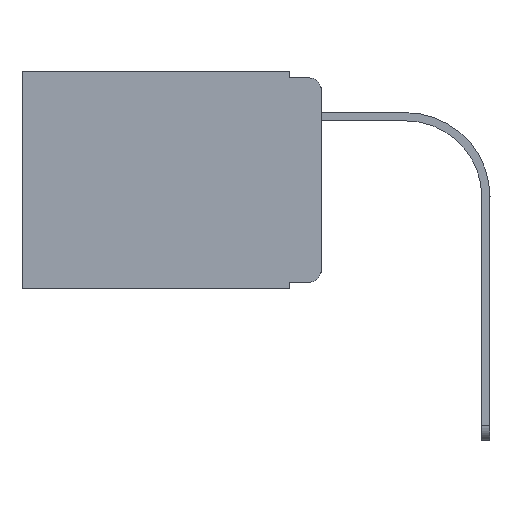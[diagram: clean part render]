
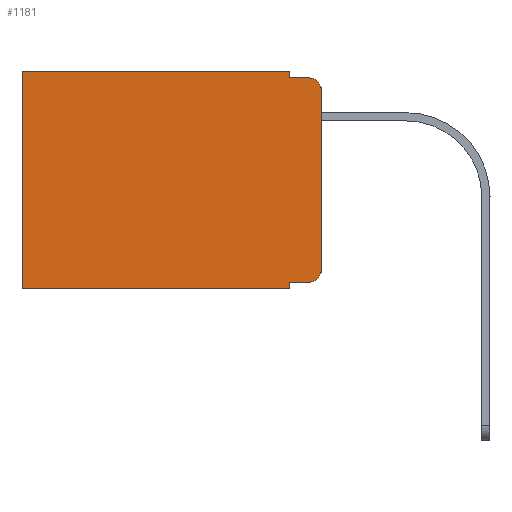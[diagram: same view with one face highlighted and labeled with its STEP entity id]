
A CAD part, left-side view. The second image highlights one B-rep face of the part: STEP entity #1181.
In plain terms, the highlighted planar face has unit normal (-1, 0, 0).
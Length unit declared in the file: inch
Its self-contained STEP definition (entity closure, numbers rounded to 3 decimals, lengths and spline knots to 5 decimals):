
#88 = DIRECTION ( 'NONE',  ( 0., 1., 0. ) ) ;
#89 = VERTEX_POINT ( 'NONE', #3949 ) ;
#189 = CARTESIAN_POINT ( 'NONE',  ( 0.298, 0., 0. ) ) ;
#239 = LINE ( 'NONE', #189, #3472 ) ;
#240 = ORIENTED_EDGE ( 'NONE', *, *, #1186, .T. ) ;
#448 = DIRECTION ( 'NONE',  ( 0., 0., -1. ) ) ;
#552 = EDGE_CURVE ( 'NONE', #5223, #10134, #5753, .T. ) ;
#951 = DIRECTION ( 'NONE',  ( -1., 0., 0. ) ) ;
#1024 = VERTEX_POINT ( 'NONE', #6915 ) ;
#1033 = FACE_OUTER_BOUND ( 'NONE', #5975, .T. ) ;
#1137 = ORIENTED_EDGE ( 'NONE', *, *, #7990, .T. ) ;
#1181 = ADVANCED_FACE ( 'NONE', ( #1033 ), #5618, .F. ) ;
#1186 = EDGE_CURVE ( 'NONE', #3363, #9292, #239, .T. ) ;
#1256 = VERTEX_POINT ( 'NONE', #2739 ) ;
#1648 = VERTEX_POINT ( 'NONE', #8376 ) ;
#1734 = VECTOR ( 'NONE', #4858, 39.37008 ) ;
#1932 = CARTESIAN_POINT ( 'NONE',  ( 0.298, 0.051, -0.333 ) ) ;
#2245 = CARTESIAN_POINT ( 'NONE',  ( 0.298, 0., 0. ) ) ;
#2311 = LINE ( 'NONE', #7768, #10085 ) ;
#2401 = VECTOR ( 'NONE', #448, 39.37008 ) ;
#2627 = CIRCLE ( 'NONE', #2946, 0.02 ) ;
#2739 = CARTESIAN_POINT ( 'NONE',  ( 0.298, 0.051, -0.343 ) ) ;
#2856 = CARTESIAN_POINT ( 'NONE',  ( 0.298, 0.473, 0. ) ) ;
#2946 = AXIS2_PLACEMENT_3D ( 'NONE', #3174, #951, #6260 ) ;
#3081 = CARTESIAN_POINT ( 'NONE',  ( 0.298, 0.02, -0.313 ) ) ;
#3103 = ORIENTED_EDGE ( 'NONE', *, *, #4603, .F. ) ;
#3139 = DIRECTION ( 'NONE',  ( 0., -1., 0. ) ) ;
#3174 = CARTESIAN_POINT ( 'NONE',  ( 0.298, 0.02, -0.03 ) ) ;
#3324 = AXIS2_PLACEMENT_3D ( 'NONE', #4110, #3389, #7936 ) ;
#3363 = VERTEX_POINT ( 'NONE', #3829 ) ;
#3389 = DIRECTION ( 'NONE',  ( 1., 0., 0. ) ) ;
#3392 = ORIENTED_EDGE ( 'NONE', *, *, #9044, .F. ) ;
#3472 = VECTOR ( 'NONE', #88, 39.37008 ) ;
#3829 = CARTESIAN_POINT ( 'NONE',  ( 0.298, 0.051, 0. ) ) ;
#3929 = VECTOR ( 'NONE', #8483, 39.37008 ) ;
#3949 = CARTESIAN_POINT ( 'NONE',  ( 0.298, 0., -0.03 ) ) ;
#4045 = CARTESIAN_POINT ( 'NONE',  ( 0.298, 0.051, -0.01 ) ) ;
#4110 = CARTESIAN_POINT ( 'NONE',  ( 0.298, 0., 0. ) ) ;
#4142 = LINE ( 'NONE', #8029, #1734 ) ;
#4181 = ORIENTED_EDGE ( 'NONE', *, *, #8760, .F. ) ;
#4237 = AXIS2_PLACEMENT_3D ( 'NONE', #3081, #7598, #8438 ) ;
#4336 = CARTESIAN_POINT ( 'NONE',  ( 0.298, 0.02, -0.333 ) ) ;
#4603 = EDGE_CURVE ( 'NONE', #5223, #1256, #7674, .T. ) ;
#4723 = VECTOR ( 'NONE', #7966, 39.37008 ) ;
#4814 = ORIENTED_EDGE ( 'NONE', *, *, #7805, .T. ) ;
#4858 = DIRECTION ( 'NONE',  ( 0., 0., -1. ) ) ;
#5137 = EDGE_CURVE ( 'NONE', #1648, #5416, #9325, .T. ) ;
#5188 = EDGE_CURVE ( 'NONE', #1256, #9279, #2311, .T. ) ;
#5223 = VERTEX_POINT ( 'NONE', #1932 ) ;
#5351 = CARTESIAN_POINT ( 'NONE',  ( 0.298, 0.02, -0.01 ) ) ;
#5413 = DIRECTION ( 'NONE',  ( 0., 1., 0. ) ) ;
#5416 = VERTEX_POINT ( 'NONE', #5351 ) ;
#5487 = VECTOR ( 'NONE', #3139, 39.37008 ) ;
#5618 = PLANE ( 'NONE',  #3324 ) ;
#5753 = LINE ( 'NONE', #9616, #4723 ) ;
#5777 = ORIENTED_EDGE ( 'NONE', *, *, #5137, .F. ) ;
#5834 = EDGE_CURVE ( 'NONE', #9292, #9279, #4142, .T. ) ;
#5862 = ORIENTED_EDGE ( 'NONE', *, *, #5834, .T. ) ;
#5975 = EDGE_LOOP ( 'NONE', ( #4181, #1137, #5777, #3392, #240, #5862, #6372, #3103, #9537, #4814 ) ) ;
#6260 = DIRECTION ( 'NONE',  ( 0., 0., -1. ) ) ;
#6372 = ORIENTED_EDGE ( 'NONE', *, *, #5188, .F. ) ;
#6747 = LINE ( 'NONE', #8305, #2401 ) ;
#6915 = CARTESIAN_POINT ( 'NONE',  ( 0.298, 0., -0.313 ) ) ;
#7524 = DIRECTION ( 'NONE',  ( 0., 0., -1. ) ) ;
#7598 = DIRECTION ( 'NONE',  ( -1., 0., 0. ) ) ;
#7617 = CARTESIAN_POINT ( 'NONE',  ( 0.298, 0.051, 0. ) ) ;
#7674 = LINE ( 'NONE', #7617, #8754 ) ;
#7768 = CARTESIAN_POINT ( 'NONE',  ( 0.298, 0., -0.343 ) ) ;
#7805 = EDGE_CURVE ( 'NONE', #10134, #1024, #8655, .T. ) ;
#7936 = DIRECTION ( 'NONE',  ( 0., 0., -1. ) ) ;
#7966 = DIRECTION ( 'NONE',  ( 0., -1., 0. ) ) ;
#7990 = EDGE_CURVE ( 'NONE', #89, #5416, #2627, .T. ) ;
#8029 = CARTESIAN_POINT ( 'NONE',  ( 0.298, 0.473, 0. ) ) ;
#8305 = CARTESIAN_POINT ( 'NONE',  ( 0.298, 0.051, 0. ) ) ;
#8376 = CARTESIAN_POINT ( 'NONE',  ( 0.298, 0.051, -0.01 ) ) ;
#8438 = DIRECTION ( 'NONE',  ( 0., 0., -1. ) ) ;
#8483 = DIRECTION ( 'NONE',  ( 0., 0., -1. ) ) ;
#8655 = CIRCLE ( 'NONE', #4237, 0.02 ) ;
#8754 = VECTOR ( 'NONE', #7524, 39.37008 ) ;
#8760 = EDGE_CURVE ( 'NONE', #89, #1024, #9208, .T. ) ;
#9044 = EDGE_CURVE ( 'NONE', #3363, #1648, #6747, .T. ) ;
#9208 = LINE ( 'NONE', #2245, #3929 ) ;
#9279 = VERTEX_POINT ( 'NONE', #9863 ) ;
#9292 = VERTEX_POINT ( 'NONE', #2856 ) ;
#9325 = LINE ( 'NONE', #4045, #5487 ) ;
#9537 = ORIENTED_EDGE ( 'NONE', *, *, #552, .T. ) ;
#9616 = CARTESIAN_POINT ( 'NONE',  ( 0.298, 0.051, -0.333 ) ) ;
#9863 = CARTESIAN_POINT ( 'NONE',  ( 0.298, 0.473, -0.343 ) ) ;
#10085 = VECTOR ( 'NONE', #5413, 39.37008 ) ;
#10134 = VERTEX_POINT ( 'NONE', #4336 ) ;
